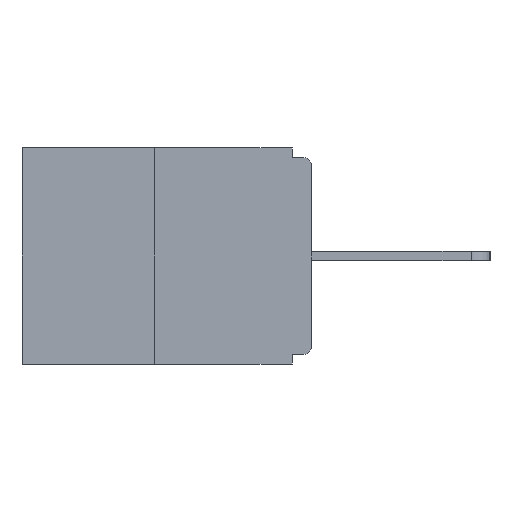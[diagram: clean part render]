
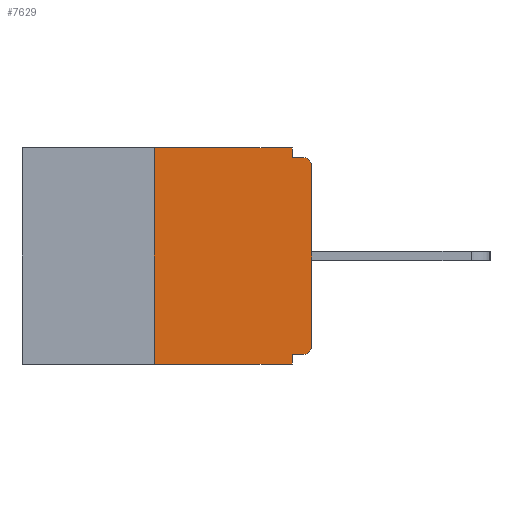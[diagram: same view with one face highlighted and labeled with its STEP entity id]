
A CAD part, left-side view. The second image highlights one B-rep face of the part: STEP entity #7629.
In plain terms, the highlighted planar face has unit normal (-1, 0, 0).
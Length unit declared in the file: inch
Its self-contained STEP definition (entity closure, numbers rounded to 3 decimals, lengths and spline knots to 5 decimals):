
#126 = LINE ( 'NONE', #9717, #10718 ) ;
#129 = DIRECTION ( 'NONE',  ( 0., 0., 1. ) ) ;
#569 = CARTESIAN_POINT ( 'NONE',  ( 0., 0.25, 0. ) ) ;
#936 = CARTESIAN_POINT ( 'NONE',  ( 0., 0.015, -0.03 ) ) ;
#952 = CIRCLE ( 'NONE', #3658, 0.015 ) ;
#1595 = LINE ( 'NONE', #8023, #3746 ) ;
#1749 = ORIENTED_EDGE ( 'NONE', *, *, #20221, .F. ) ;
#2068 = DIRECTION ( 'NONE',  ( 1., 0., 0. ) ) ;
#2190 = EDGE_CURVE ( 'NONE', #19996, #3541, #4382, .T. ) ;
#2363 = VECTOR ( 'NONE', #8242, 39.37008 ) ;
#2504 = EDGE_CURVE ( 'NONE', #8952, #9158, #5188, .T. ) ;
#2594 = CARTESIAN_POINT ( 'NONE',  ( 0., 0., -0.015 ) ) ;
#2788 = DIRECTION ( 'NONE',  ( 0., -1., 0. ) ) ;
#2863 = LINE ( 'NONE', #4776, #4412 ) ;
#3541 = VERTEX_POINT ( 'NONE', #5823 ) ;
#3649 = DIRECTION ( 'NONE',  ( 0., 0., -1. ) ) ;
#3658 = AXIS2_PLACEMENT_3D ( 'NONE', #19217, #14467, #11070 ) ;
#3721 = EDGE_LOOP ( 'NONE', ( #19275, #18415, #14243, #1749, #18341, #7833, #16107, #8302, #13332, #6516 ) ) ;
#3746 = VECTOR ( 'NONE', #129, 39.37008 ) ;
#3856 = EDGE_CURVE ( 'NONE', #16670, #9158, #6086, .T. ) ;
#4382 = LINE ( 'NONE', #20830, #7182 ) ;
#4412 = VECTOR ( 'NONE', #15739, 39.37008 ) ;
#4776 = CARTESIAN_POINT ( 'NONE',  ( 0., 0.031, 0. ) ) ;
#4875 = DIRECTION ( 'NONE',  ( 0., 0., 1. ) ) ;
#4931 = EDGE_CURVE ( 'NONE', #19996, #9218, #126, .T. ) ;
#5188 = CIRCLE ( 'NONE', #16968, 0.015 ) ;
#5251 = VERTEX_POINT ( 'NONE', #17614 ) ;
#5488 = EDGE_CURVE ( 'NONE', #19222, #9048, #18833, .T. ) ;
#5823 = CARTESIAN_POINT ( 'NONE',  ( 0., 0.031, -0.343 ) ) ;
#6036 = EDGE_CURVE ( 'NONE', #5251, #16670, #2863, .T. ) ;
#6086 = LINE ( 'NONE', #2594, #12955 ) ;
#6516 = ORIENTED_EDGE ( 'NONE', *, *, #6036, .F. ) ;
#6716 = CARTESIAN_POINT ( 'NONE',  ( 0., 0.46, 0. ) ) ;
#7182 = VECTOR ( 'NONE', #2788, 39.37008 ) ;
#7280 = DIRECTION ( 'NONE',  ( 0., 0., -1. ) ) ;
#7540 = CARTESIAN_POINT ( 'NONE',  ( 0., 0.031, -0.343 ) ) ;
#7629 = ADVANCED_FACE ( 'NONE', ( #19605 ), #11462, .F. ) ;
#7833 = ORIENTED_EDGE ( 'NONE', *, *, #9875, .T. ) ;
#8023 = CARTESIAN_POINT ( 'NONE',  ( 0., 0., 0. ) ) ;
#8242 = DIRECTION ( 'NONE',  ( 0., -1., 0. ) ) ;
#8302 = ORIENTED_EDGE ( 'NONE', *, *, #2504, .T. ) ;
#8952 = VERTEX_POINT ( 'NONE', #20228 ) ;
#9048 = VERTEX_POINT ( 'NONE', #11331 ) ;
#9158 = VERTEX_POINT ( 'NONE', #15882 ) ;
#9218 = VERTEX_POINT ( 'NONE', #569 ) ;
#9717 = CARTESIAN_POINT ( 'NONE',  ( 0., 0.25, 0. ) ) ;
#9875 = EDGE_CURVE ( 'NONE', #19222, #19614, #952, .T. ) ;
#10653 = DIRECTION ( 'NONE',  ( -1., 0., 0. ) ) ;
#10718 = VECTOR ( 'NONE', #4875, 39.37008 ) ;
#11070 = DIRECTION ( 'NONE',  ( 0., 0., -1. ) ) ;
#11331 = CARTESIAN_POINT ( 'NONE',  ( 0., 0.031, -0.328 ) ) ;
#11439 = VECTOR ( 'NONE', #20629, 39.37008 ) ;
#11462 = PLANE ( 'NONE',  #19212 ) ;
#12174 = CARTESIAN_POINT ( 'NONE',  ( 0., 0.031, -0.015 ) ) ;
#12487 = CARTESIAN_POINT ( 'NONE',  ( 0., 0.015, -0.328 ) ) ;
#12516 = VECTOR ( 'NONE', #13895, 39.37008 ) ;
#12955 = VECTOR ( 'NONE', #17263, 39.37008 ) ;
#13083 = EDGE_CURVE ( 'NONE', #19614, #8952, #1595, .T. ) ;
#13332 = ORIENTED_EDGE ( 'NONE', *, *, #3856, .F. ) ;
#13895 = DIRECTION ( 'NONE',  ( 0., 1., 0. ) ) ;
#14243 = ORIENTED_EDGE ( 'NONE', *, *, #2190, .T. ) ;
#14467 = DIRECTION ( 'NONE',  ( -1., 0., 0. ) ) ;
#15449 = CARTESIAN_POINT ( 'NONE',  ( 0., 0., -0.328 ) ) ;
#15739 = DIRECTION ( 'NONE',  ( 0., 0., -1. ) ) ;
#15871 = LINE ( 'NONE', #7540, #11439 ) ;
#15882 = CARTESIAN_POINT ( 'NONE',  ( 0., 0.015, -0.015 ) ) ;
#16107 = ORIENTED_EDGE ( 'NONE', *, *, #13083, .T. ) ;
#16208 = CARTESIAN_POINT ( 'NONE',  ( 0., 0.25, -0.343 ) ) ;
#16670 = VERTEX_POINT ( 'NONE', #12174 ) ;
#16968 = AXIS2_PLACEMENT_3D ( 'NONE', #936, #10653, #7280 ) ;
#17263 = DIRECTION ( 'NONE',  ( 0., -1., 0. ) ) ;
#17614 = CARTESIAN_POINT ( 'NONE',  ( 0., 0.031, 0. ) ) ;
#17849 = CARTESIAN_POINT ( 'NONE',  ( 0., 0.46, 0. ) ) ;
#18341 = ORIENTED_EDGE ( 'NONE', *, *, #5488, .F. ) ;
#18415 = ORIENTED_EDGE ( 'NONE', *, *, #4931, .F. ) ;
#18833 = LINE ( 'NONE', #15449, #12516 ) ;
#19119 = LINE ( 'NONE', #17849, #2363 ) ;
#19212 = AXIS2_PLACEMENT_3D ( 'NONE', #6716, #2068, #3649 ) ;
#19217 = CARTESIAN_POINT ( 'NONE',  ( 0., 0.015, -0.313 ) ) ;
#19222 = VERTEX_POINT ( 'NONE', #12487 ) ;
#19275 = ORIENTED_EDGE ( 'NONE', *, *, #20763, .F. ) ;
#19543 = CARTESIAN_POINT ( 'NONE',  ( 0., 0., -0.313 ) ) ;
#19605 = FACE_OUTER_BOUND ( 'NONE', #3721, .T. ) ;
#19614 = VERTEX_POINT ( 'NONE', #19543 ) ;
#19996 = VERTEX_POINT ( 'NONE', #16208 ) ;
#20221 = EDGE_CURVE ( 'NONE', #9048, #3541, #15871, .T. ) ;
#20228 = CARTESIAN_POINT ( 'NONE',  ( 0., 0., -0.03 ) ) ;
#20629 = DIRECTION ( 'NONE',  ( 0., 0., -1. ) ) ;
#20763 = EDGE_CURVE ( 'NONE', #9218, #5251, #19119, .T. ) ;
#20830 = CARTESIAN_POINT ( 'NONE',  ( 0., 0.46, -0.343 ) ) ;
